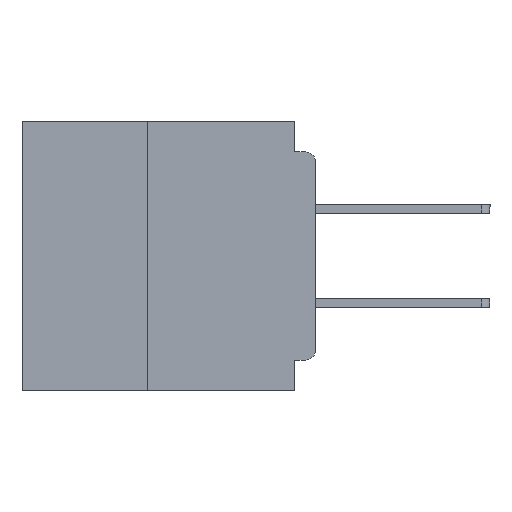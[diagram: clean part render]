
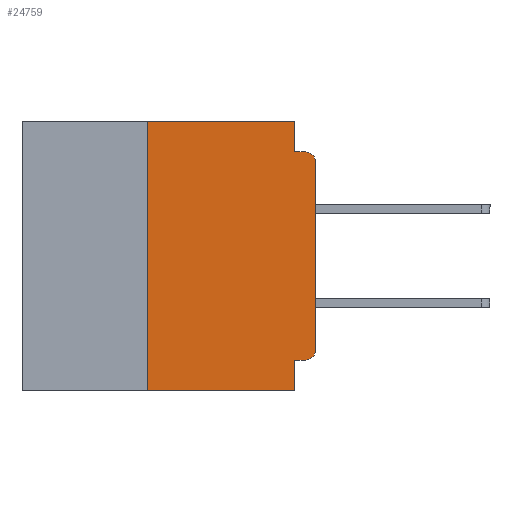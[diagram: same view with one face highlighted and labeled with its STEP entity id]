
A CAD part, left-side view. The second image highlights one B-rep face of the part: STEP entity #24759.
In plain terms, the highlighted planar face has unit normal (-1, 0, 0).
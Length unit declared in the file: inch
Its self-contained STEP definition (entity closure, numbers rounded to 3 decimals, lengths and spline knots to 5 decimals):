
#1159 = DIRECTION ( 'NONE',  ( 0., 0., -1. ) ) ;
#2412 = LINE ( 'NONE', #45682, #12883 ) ;
#2502 = CARTESIAN_POINT ( 'NONE',  ( 0., 0., -0.34 ) ) ;
#2795 = ORIENTED_EDGE ( 'NONE', *, *, #49892, .T. ) ;
#3479 = ORIENTED_EDGE ( 'NONE', *, *, #41555, .F. ) ;
#3801 = EDGE_CURVE ( 'NONE', #45226, #32562, #21530, .T. ) ;
#5559 = LINE ( 'NONE', #47719, #18873 ) ;
#6351 = LINE ( 'NONE', #39478, #18282 ) ;
#7047 = VECTOR ( 'NONE', #7209, 39.37008 ) ;
#7209 = DIRECTION ( 'NONE',  ( 0., 1., 0. ) ) ;
#8516 = EDGE_CURVE ( 'NONE', #45226, #14776, #52470, .T. ) ;
#9323 = DIRECTION ( 'NONE',  ( -1., 0., 0. ) ) ;
#9505 = AXIS2_PLACEMENT_3D ( 'NONE', #14402, #27954, #1159 ) ;
#9620 = EDGE_CURVE ( 'NONE', #56610, #30174, #53022, .T. ) ;
#9825 = CARTESIAN_POINT ( 'NONE',  ( 0., 0.031, 0. ) ) ;
#10290 = DIRECTION ( 'NONE',  ( 0., -1., 0. ) ) ;
#10581 = EDGE_CURVE ( 'NONE', #52184, #57704, #17438, .T. ) ;
#11246 = FACE_OUTER_BOUND ( 'NONE', #35372, .T. ) ;
#11859 = AXIS2_PLACEMENT_3D ( 'NONE', #47935, #21342, #52400 ) ;
#12728 = DIRECTION ( 'NONE',  ( 0., 0., -1. ) ) ;
#12883 = VECTOR ( 'NONE', #50179, 39.37008 ) ;
#13264 = CARTESIAN_POINT ( 'NONE',  ( 0., 0.015, -0.045 ) ) ;
#14402 = CARTESIAN_POINT ( 'NONE',  ( 0., 0.437, 0. ) ) ;
#14776 = VERTEX_POINT ( 'NONE', #56756 ) ;
#15075 = CARTESIAN_POINT ( 'NONE',  ( 0., 0., -0.06 ) ) ;
#15393 = ORIENTED_EDGE ( 'NONE', *, *, #18885, .F. ) ;
#16523 = ORIENTED_EDGE ( 'NONE', *, *, #9620, .F. ) ;
#17438 = LINE ( 'NONE', #9825, #50124 ) ;
#18282 = VECTOR ( 'NONE', #12728, 39.37008 ) ;
#18730 = CARTESIAN_POINT ( 'NONE',  ( 0., 0.031, -0.045 ) ) ;
#18873 = VECTOR ( 'NONE', #52193, 39.37008 ) ;
#18885 = EDGE_CURVE ( 'NONE', #57704, #26486, #53853, .T. ) ;
#19788 = EDGE_CURVE ( 'NONE', #30174, #32562, #6351, .T. ) ;
#19803 = VECTOR ( 'NONE', #10290, 39.37008 ) ;
#20317 = CIRCLE ( 'NONE', #53181, 0.015 ) ;
#20782 = ORIENTED_EDGE ( 'NONE', *, *, #36260, .T. ) ;
#21342 = DIRECTION ( 'NONE',  ( -1., 0., 0. ) ) ;
#21530 = LINE ( 'NONE', #52372, #29166 ) ;
#23693 = CARTESIAN_POINT ( 'NONE',  ( 0., 0.031, -0.355 ) ) ;
#24215 = VERTEX_POINT ( 'NONE', #15075 ) ;
#24759 = ADVANCED_FACE ( 'NONE', ( #11246 ), #41178, .F. ) ;
#25264 = EDGE_CURVE ( 'NONE', #24215, #26486, #20317, .T. ) ;
#26349 = DIRECTION ( 'NONE',  ( 0., 0., 1. ) ) ;
#26486 = VERTEX_POINT ( 'NONE', #13264 ) ;
#27615 = DIRECTION ( 'NONE',  ( 0., 0., -1. ) ) ;
#27954 = DIRECTION ( 'NONE',  ( 1., 0., 0. ) ) ;
#29166 = VECTOR ( 'NONE', #30261, 39.37008 ) ;
#30174 = VERTEX_POINT ( 'NONE', #23693 ) ;
#30261 = DIRECTION ( 'NONE',  ( 0., -1., 0. ) ) ;
#32562 = VERTEX_POINT ( 'NONE', #43019 ) ;
#33677 = CARTESIAN_POINT ( 'NONE',  ( 0., 0.015, -0.355 ) ) ;
#34718 = CARTESIAN_POINT ( 'NONE',  ( 0., 0.031, 0. ) ) ;
#35372 = EDGE_LOOP ( 'NONE', ( #20782, #52280, #15393, #46748, #3479, #39559, #52461, #46022, #16523, #2795 ) ) ;
#36045 = CARTESIAN_POINT ( 'NONE',  ( 0., 0.015, -0.06 ) ) ;
#36260 = EDGE_CURVE ( 'NONE', #42887, #24215, #5559, .T. ) ;
#37015 = CARTESIAN_POINT ( 'NONE',  ( 0., 0., -0.045 ) ) ;
#39478 = CARTESIAN_POINT ( 'NONE',  ( 0., 0.031, -0.4 ) ) ;
#39559 = ORIENTED_EDGE ( 'NONE', *, *, #8516, .F. ) ;
#39580 = CARTESIAN_POINT ( 'NONE',  ( 0., 0.25, -0.4 ) ) ;
#40531 = DIRECTION ( 'NONE',  ( 0., 0., -1. ) ) ;
#41043 = CIRCLE ( 'NONE', #11859, 0.015 ) ;
#41178 = PLANE ( 'NONE',  #9505 ) ;
#41555 = EDGE_CURVE ( 'NONE', #14776, #52184, #2412, .T. ) ;
#42871 = CARTESIAN_POINT ( 'NONE',  ( 0., 0., -0.355 ) ) ;
#42887 = VERTEX_POINT ( 'NONE', #2502 ) ;
#43019 = CARTESIAN_POINT ( 'NONE',  ( 0., 0.031, -0.4 ) ) ;
#45226 = VERTEX_POINT ( 'NONE', #53461 ) ;
#45682 = CARTESIAN_POINT ( 'NONE',  ( 0., 0.437, 0. ) ) ;
#46022 = ORIENTED_EDGE ( 'NONE', *, *, #19788, .F. ) ;
#46748 = ORIENTED_EDGE ( 'NONE', *, *, #10581, .F. ) ;
#47719 = CARTESIAN_POINT ( 'NONE',  ( 0., 0., 0. ) ) ;
#47935 = CARTESIAN_POINT ( 'NONE',  ( 0., 0.015, -0.34 ) ) ;
#49892 = EDGE_CURVE ( 'NONE', #56610, #42887, #41043, .T. ) ;
#50124 = VECTOR ( 'NONE', #27615, 39.37008 ) ;
#50179 = DIRECTION ( 'NONE',  ( 0., -1., 0. ) ) ;
#51076 = VECTOR ( 'NONE', #26349, 39.37008 ) ;
#52184 = VERTEX_POINT ( 'NONE', #34718 ) ;
#52193 = DIRECTION ( 'NONE',  ( 0., 0., 1. ) ) ;
#52280 = ORIENTED_EDGE ( 'NONE', *, *, #25264, .T. ) ;
#52372 = CARTESIAN_POINT ( 'NONE',  ( 0., 0.437, -0.4 ) ) ;
#52400 = DIRECTION ( 'NONE',  ( 0., 0., -1. ) ) ;
#52461 = ORIENTED_EDGE ( 'NONE', *, *, #3801, .T. ) ;
#52470 = LINE ( 'NONE', #39580, #51076 ) ;
#53022 = LINE ( 'NONE', #42871, #7047 ) ;
#53181 = AXIS2_PLACEMENT_3D ( 'NONE', #36045, #9323, #40531 ) ;
#53461 = CARTESIAN_POINT ( 'NONE',  ( 0., 0.25, -0.4 ) ) ;
#53853 = LINE ( 'NONE', #37015, #19803 ) ;
#56610 = VERTEX_POINT ( 'NONE', #33677 ) ;
#56756 = CARTESIAN_POINT ( 'NONE',  ( 0., 0.25, 0. ) ) ;
#57704 = VERTEX_POINT ( 'NONE', #18730 ) ;
